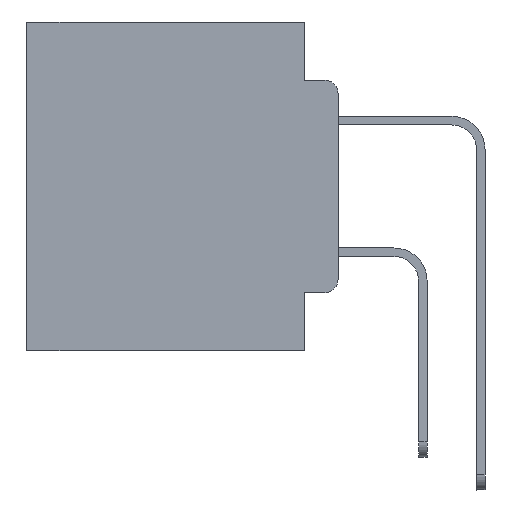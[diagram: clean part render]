
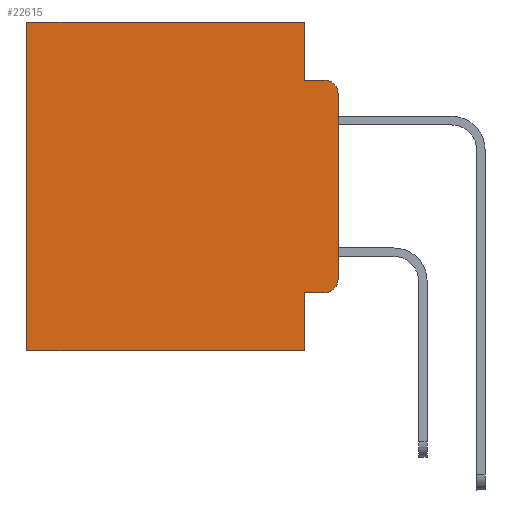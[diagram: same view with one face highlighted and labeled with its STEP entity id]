
A CAD part, left-side view. The second image highlights one B-rep face of the part: STEP entity #22615.
In plain terms, the highlighted planar face has unit normal (-1, 0, 0).
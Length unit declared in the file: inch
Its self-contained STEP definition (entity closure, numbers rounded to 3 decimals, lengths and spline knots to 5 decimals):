
#431 = CARTESIAN_POINT ( 'NONE',  ( 0.298, 0., 0. ) ) ;
#470 = DIRECTION ( 'NONE',  ( 0., 0., -1. ) ) ;
#708 = LINE ( 'NONE', #431, #7213 ) ;
#2589 = CARTESIAN_POINT ( 'NONE',  ( 0.298, 0.051, -0.0885 ) ) ;
#3056 = EDGE_CURVE ( 'NONE', #7135, #3360, #21049, .T. ) ;
#3360 = VERTEX_POINT ( 'NONE', #23876 ) ;
#3410 = CARTESIAN_POINT ( 'NONE',  ( 0.298, 0.02, -0.3915 ) ) ;
#3799 = LINE ( 'NONE', #16250, #25559 ) ;
#3926 = ORIENTED_EDGE ( 'NONE', *, *, #10533, .F. ) ;
#4608 = VECTOR ( 'NONE', #22558, 39.37008 ) ;
#5247 = ORIENTED_EDGE ( 'NONE', *, *, #17072, .T. ) ;
#5552 = DIRECTION ( 'NONE',  ( 0., 0., -1. ) ) ;
#6018 = VECTOR ( 'NONE', #18674, 39.37008 ) ;
#6922 = CARTESIAN_POINT ( 'NONE',  ( 0.298, 0.02, -0.0885 ) ) ;
#7135 = VERTEX_POINT ( 'NONE', #16353 ) ;
#7213 = VECTOR ( 'NONE', #15554, 39.37008 ) ;
#7281 = ORIENTED_EDGE ( 'NONE', *, *, #3056, .T. ) ;
#7729 = LINE ( 'NONE', #21589, #12783 ) ;
#7748 = CARTESIAN_POINT ( 'NONE',  ( 0.298, 0.473, -0.5 ) ) ;
#8458 = AXIS2_PLACEMENT_3D ( 'NONE', #9774, #24300, #11919 ) ;
#8547 = AXIS2_PLACEMENT_3D ( 'NONE', #23299, #10924, #25395 ) ;
#9052 = EDGE_CURVE ( 'NONE', #16777, #9165, #3799, .T. ) ;
#9075 = ORIENTED_EDGE ( 'NONE', *, *, #10831, .T. ) ;
#9165 = VERTEX_POINT ( 'NONE', #12483 ) ;
#9774 = CARTESIAN_POINT ( 'NONE',  ( 0.298, 0., 0. ) ) ;
#10101 = ORIENTED_EDGE ( 'NONE', *, *, #9052, .F. ) ;
#10107 = VERTEX_POINT ( 'NONE', #24439 ) ;
#10533 = EDGE_CURVE ( 'NONE', #9165, #15522, #7729, .T. ) ;
#10551 = VERTEX_POINT ( 'NONE', #6922 ) ;
#10831 = EDGE_CURVE ( 'NONE', #21210, #10107, #16043, .T. ) ;
#10924 = DIRECTION ( 'NONE',  ( -1., 0., 0. ) ) ;
#11197 = EDGE_CURVE ( 'NONE', #21210, #24138, #12406, .T. ) ;
#11216 = VECTOR ( 'NONE', #24179, 39.37008 ) ;
#11803 = LINE ( 'NONE', #24721, #6018 ) ;
#11919 = DIRECTION ( 'NONE',  ( 0., 0., -1. ) ) ;
#12215 = CARTESIAN_POINT ( 'NONE',  ( 0.298, 0., 0. ) ) ;
#12406 = LINE ( 'NONE', #19786, #16666 ) ;
#12483 = CARTESIAN_POINT ( 'NONE',  ( 0.298, 0.051, -0.5 ) ) ;
#12783 = VECTOR ( 'NONE', #13323, 39.37008 ) ;
#12815 = VECTOR ( 'NONE', #5552, 39.37008 ) ;
#12961 = VERTEX_POINT ( 'NONE', #17566 ) ;
#12988 = EDGE_CURVE ( 'NONE', #12961, #3360, #708, .T. ) ;
#13323 = DIRECTION ( 'NONE',  ( 0., 1., 0. ) ) ;
#13861 = DIRECTION ( 'NONE',  ( -1., 0., 0. ) ) ;
#14628 = CIRCLE ( 'NONE', #8547, 0.02 ) ;
#15522 = VERTEX_POINT ( 'NONE', #7748 ) ;
#15554 = DIRECTION ( 'NONE',  ( 0., 0., -1. ) ) ;
#16043 = LINE ( 'NONE', #12215, #4608 ) ;
#16250 = CARTESIAN_POINT ( 'NONE',  ( 0.298, 0.051, 0. ) ) ;
#16353 = CARTESIAN_POINT ( 'NONE',  ( 0.298, 0.02, -0.4115 ) ) ;
#16666 = VECTOR ( 'NONE', #470, 39.37008 ) ;
#16777 = VERTEX_POINT ( 'NONE', #26379 ) ;
#16939 = EDGE_LOOP ( 'NONE', ( #25619, #5247, #17337, #27334, #9075, #18297, #3926, #10101, #19570, #7281 ) ) ;
#17072 = EDGE_CURVE ( 'NONE', #12961, #10551, #14628, .T. ) ;
#17337 = ORIENTED_EDGE ( 'NONE', *, *, #20910, .F. ) ;
#17398 = CARTESIAN_POINT ( 'NONE',  ( 0.298, 0.051, 0. ) ) ;
#17428 = LINE ( 'NONE', #22152, #11216 ) ;
#17566 = CARTESIAN_POINT ( 'NONE',  ( 0.298, 0., -0.1085 ) ) ;
#18297 = ORIENTED_EDGE ( 'NONE', *, *, #23855, .T. ) ;
#18357 = DIRECTION ( 'NONE',  ( 0., 0., -1. ) ) ;
#18674 = DIRECTION ( 'NONE',  ( 0., -1., 0. ) ) ;
#18809 = DIRECTION ( 'NONE',  ( 0., 0., -1. ) ) ;
#19570 = ORIENTED_EDGE ( 'NONE', *, *, #23231, .T. ) ;
#19786 = CARTESIAN_POINT ( 'NONE',  ( 0.298, 0.051, 0. ) ) ;
#20062 = FACE_OUTER_BOUND ( 'NONE', #16939, .T. ) ;
#20910 = EDGE_CURVE ( 'NONE', #24138, #10551, #11803, .T. ) ;
#21049 = CIRCLE ( 'NONE', #26963, 0.02 ) ;
#21210 = VERTEX_POINT ( 'NONE', #17398 ) ;
#21589 = CARTESIAN_POINT ( 'NONE',  ( 0.298, 0., -0.5 ) ) ;
#22152 = CARTESIAN_POINT ( 'NONE',  ( 0.298, 0.051, -0.4115 ) ) ;
#22273 = PLANE ( 'NONE',  #8458 ) ;
#22558 = DIRECTION ( 'NONE',  ( 0., 1., 0. ) ) ;
#22615 = ADVANCED_FACE ( 'NONE', ( #20062 ), #22273, .F. ) ;
#23231 = EDGE_CURVE ( 'NONE', #16777, #7135, #17428, .T. ) ;
#23299 = CARTESIAN_POINT ( 'NONE',  ( 0.298, 0.02, -0.1085 ) ) ;
#23855 = EDGE_CURVE ( 'NONE', #10107, #15522, #24424, .T. ) ;
#23876 = CARTESIAN_POINT ( 'NONE',  ( 0.298, 0., -0.3915 ) ) ;
#24138 = VERTEX_POINT ( 'NONE', #2589 ) ;
#24179 = DIRECTION ( 'NONE',  ( 0., -1., 0. ) ) ;
#24300 = DIRECTION ( 'NONE',  ( 1., 0., 0. ) ) ;
#24390 = CARTESIAN_POINT ( 'NONE',  ( 0.298, 0.473, 0. ) ) ;
#24424 = LINE ( 'NONE', #24390, #12815 ) ;
#24439 = CARTESIAN_POINT ( 'NONE',  ( 0.298, 0.473, 0. ) ) ;
#24721 = CARTESIAN_POINT ( 'NONE',  ( 0.298, 0.051, -0.0885 ) ) ;
#25395 = DIRECTION ( 'NONE',  ( 0., 0., -1. ) ) ;
#25559 = VECTOR ( 'NONE', #18357, 39.37008 ) ;
#25619 = ORIENTED_EDGE ( 'NONE', *, *, #12988, .F. ) ;
#26379 = CARTESIAN_POINT ( 'NONE',  ( 0.298, 0.051, -0.4115 ) ) ;
#26963 = AXIS2_PLACEMENT_3D ( 'NONE', #3410, #13861, #18809 ) ;
#27334 = ORIENTED_EDGE ( 'NONE', *, *, #11197, .F. ) ;
